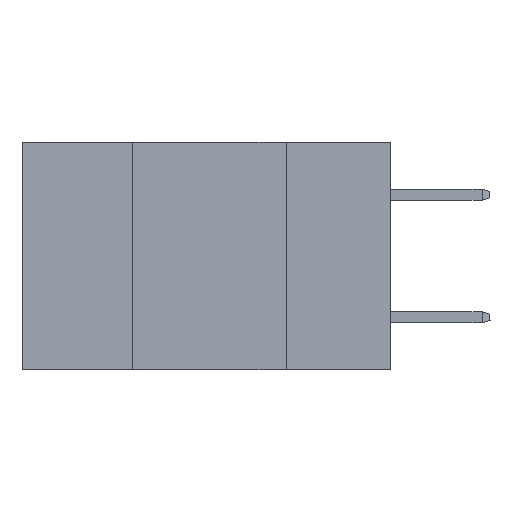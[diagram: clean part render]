
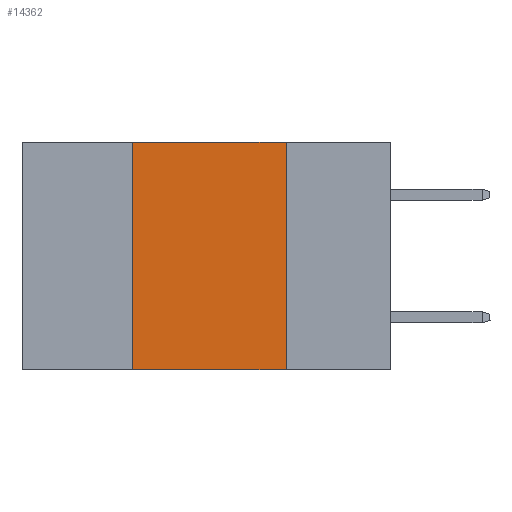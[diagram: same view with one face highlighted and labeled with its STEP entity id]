
A CAD part, left-side view. The second image highlights one B-rep face of the part: STEP entity #14362.
In plain terms, the highlighted planar face has unit normal (-1, 0, 0).
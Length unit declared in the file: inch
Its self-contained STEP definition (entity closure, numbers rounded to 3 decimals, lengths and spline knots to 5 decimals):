
#491 = CARTESIAN_POINT ( 'NONE',  ( 0., 0.42, 0. ) ) ;
#546 = CARTESIAN_POINT ( 'NONE',  ( 0., 0.17, 0. ) ) ;
#1271 = VECTOR ( 'NONE', #12446, 39.37008 ) ;
#1814 = CARTESIAN_POINT ( 'NONE',  ( 0., 0.6, 0. ) ) ;
#2159 = CARTESIAN_POINT ( 'NONE',  ( 0., 0.42, 0. ) ) ;
#3035 = LINE ( 'NONE', #6334, #18248 ) ;
#3120 = LINE ( 'NONE', #9072, #8753 ) ;
#3307 = LINE ( 'NONE', #491, #18138 ) ;
#4649 = PLANE ( 'NONE',  #18274 ) ;
#4732 = EDGE_LOOP ( 'NONE', ( #15315, #12483, #10396, #16508 ) ) ;
#4734 = DIRECTION ( 'NONE',  ( 0., -1., 0. ) ) ;
#6110 = EDGE_CURVE ( 'NONE', #8069, #15220, #3120, .T. ) ;
#6334 = CARTESIAN_POINT ( 'NONE',  ( 0., 0.6, -0.37 ) ) ;
#7062 = VERTEX_POINT ( 'NONE', #7234 ) ;
#7234 = CARTESIAN_POINT ( 'NONE',  ( 0., 0.17, -0.37 ) ) ;
#8033 = EDGE_CURVE ( 'NONE', #15220, #7062, #15089, .T. ) ;
#8069 = VERTEX_POINT ( 'NONE', #2159 ) ;
#8753 = VECTOR ( 'NONE', #4734, 39.37008 ) ;
#8803 = DIRECTION ( 'NONE',  ( 0., -1., 0. ) ) ;
#8995 = EDGE_CURVE ( 'NONE', #15340, #8069, #3307, .T. ) ;
#9072 = CARTESIAN_POINT ( 'NONE',  ( 0., 0.6, 0. ) ) ;
#10396 = ORIENTED_EDGE ( 'NONE', *, *, #8995, .F. ) ;
#11039 = CARTESIAN_POINT ( 'NONE',  ( 0., 0.17, 0. ) ) ;
#11832 = FACE_OUTER_BOUND ( 'NONE', #4732, .T. ) ;
#12446 = DIRECTION ( 'NONE',  ( 0., 0., -1. ) ) ;
#12483 = ORIENTED_EDGE ( 'NONE', *, *, #6110, .F. ) ;
#13079 = EDGE_CURVE ( 'NONE', #15340, #7062, #3035, .T. ) ;
#13786 = DIRECTION ( 'NONE',  ( 0., 0., 1. ) ) ;
#13841 = CARTESIAN_POINT ( 'NONE',  ( 0., 0.42, -0.37 ) ) ;
#14362 = ADVANCED_FACE ( 'NONE', ( #11832 ), #4649, .F. ) ;
#15089 = LINE ( 'NONE', #11039, #1271 ) ;
#15220 = VERTEX_POINT ( 'NONE', #546 ) ;
#15315 = ORIENTED_EDGE ( 'NONE', *, *, #8033, .F. ) ;
#15340 = VERTEX_POINT ( 'NONE', #13841 ) ;
#16250 = DIRECTION ( 'NONE',  ( 1., 0., 0. ) ) ;
#16508 = ORIENTED_EDGE ( 'NONE', *, *, #13079, .T. ) ;
#17773 = DIRECTION ( 'NONE',  ( 0., 0., -1. ) ) ;
#18138 = VECTOR ( 'NONE', #13786, 39.37008 ) ;
#18248 = VECTOR ( 'NONE', #8803, 39.37008 ) ;
#18274 = AXIS2_PLACEMENT_3D ( 'NONE', #1814, #16250, #17773 ) ;
